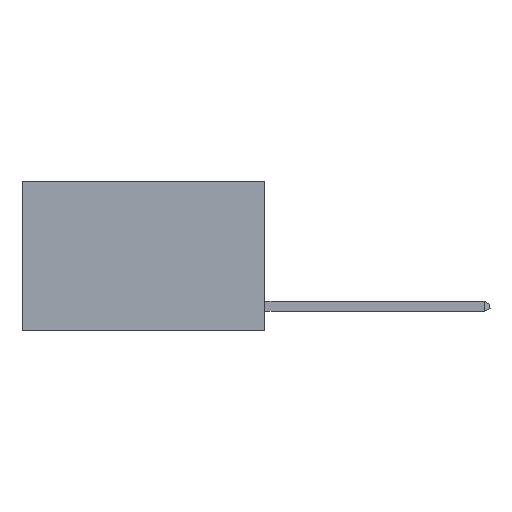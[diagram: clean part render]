
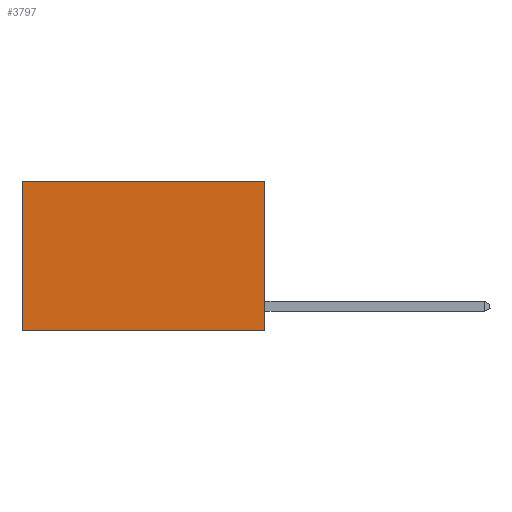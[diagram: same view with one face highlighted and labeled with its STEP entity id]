
A CAD part, left-side view. The second image highlights one B-rep face of the part: STEP entity #3797.
In plain terms, the highlighted planar face has unit normal (-1, 0, 0).
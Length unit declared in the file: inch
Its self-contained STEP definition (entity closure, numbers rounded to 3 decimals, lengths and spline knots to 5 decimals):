
#22 = LINE ( 'NONE', #12585, #5008 ) ;
#482 = VERTEX_POINT ( 'NONE', #11636 ) ;
#2139 = DIRECTION ( 'NONE',  ( 1., 0., 0. ) ) ;
#2271 = EDGE_CURVE ( 'NONE', #482, #13879, #14444, .T. ) ;
#2332 = CARTESIAN_POINT ( 'NONE',  ( 0.2625, 0., 0. ) ) ;
#2514 = AXIS2_PLACEMENT_3D ( 'NONE', #2332, #2139, #3950 ) ;
#2683 = LINE ( 'NONE', #19458, #11042 ) ;
#2715 = ORIENTED_EDGE ( 'NONE', *, *, #9157, .T. ) ;
#3133 = ORIENTED_EDGE ( 'NONE', *, *, #19628, .T. ) ;
#3490 = VECTOR ( 'NONE', #17679, 39.37008 ) ;
#3797 = ADVANCED_FACE ( 'NONE', ( #10028 ), #5564, .F. ) ;
#3950 = DIRECTION ( 'NONE',  ( 0., 0., -1. ) ) ;
#5008 = VECTOR ( 'NONE', #14102, 39.37008 ) ;
#5347 = CARTESIAN_POINT ( 'NONE',  ( 0.2625, 0., -0.37 ) ) ;
#5564 = PLANE ( 'NONE',  #2514 ) ;
#7865 = ORIENTED_EDGE ( 'NONE', *, *, #2271, .F. ) ;
#8728 = CARTESIAN_POINT ( 'NONE',  ( 0.2625, 0.6, -0.37 ) ) ;
#9157 = EDGE_CURVE ( 'NONE', #17573, #10421, #2683, .T. ) ;
#9398 = LINE ( 'NONE', #11006, #18801 ) ;
#9505 = DIRECTION ( 'NONE',  ( 0., 0., -1. ) ) ;
#10028 = FACE_OUTER_BOUND ( 'NONE', #17194, .T. ) ;
#10421 = VERTEX_POINT ( 'NONE', #19599 ) ;
#10758 = CARTESIAN_POINT ( 'NONE',  ( 0.2625, 0., 0. ) ) ;
#11006 = CARTESIAN_POINT ( 'NONE',  ( 0.2625, 0.6, 0. ) ) ;
#11042 = VECTOR ( 'NONE', #17848, 39.37008 ) ;
#11636 = CARTESIAN_POINT ( 'NONE',  ( 0.2625, 0., -0.37 ) ) ;
#12585 = CARTESIAN_POINT ( 'NONE',  ( 0.2625, 0., 0. ) ) ;
#13278 = ORIENTED_EDGE ( 'NONE', *, *, #17559, .F. ) ;
#13879 = VERTEX_POINT ( 'NONE', #8728 ) ;
#14102 = DIRECTION ( 'NONE',  ( 0., 0., -1. ) ) ;
#14444 = LINE ( 'NONE', #5347, #3490 ) ;
#17194 = EDGE_LOOP ( 'NONE', ( #3133, #7865, #13278, #2715 ) ) ;
#17559 = EDGE_CURVE ( 'NONE', #17573, #482, #22, .T. ) ;
#17573 = VERTEX_POINT ( 'NONE', #10758 ) ;
#17679 = DIRECTION ( 'NONE',  ( 0., 1., 0. ) ) ;
#17848 = DIRECTION ( 'NONE',  ( 0., 1., 0. ) ) ;
#18801 = VECTOR ( 'NONE', #9505, 39.37008 ) ;
#19458 = CARTESIAN_POINT ( 'NONE',  ( 0.2625, 0., 0. ) ) ;
#19599 = CARTESIAN_POINT ( 'NONE',  ( 0.2625, 0.6, 0. ) ) ;
#19628 = EDGE_CURVE ( 'NONE', #10421, #13879, #9398, .T. ) ;
